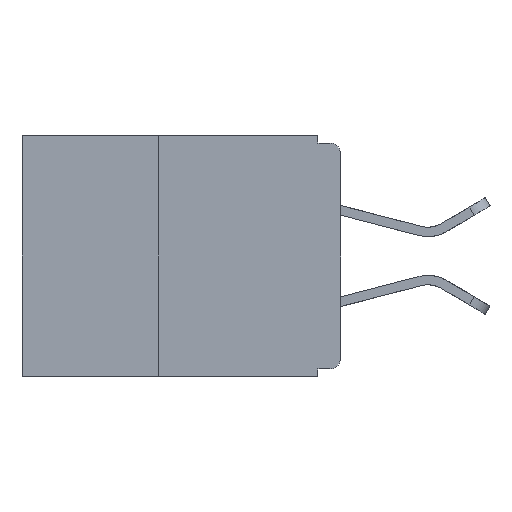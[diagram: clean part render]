
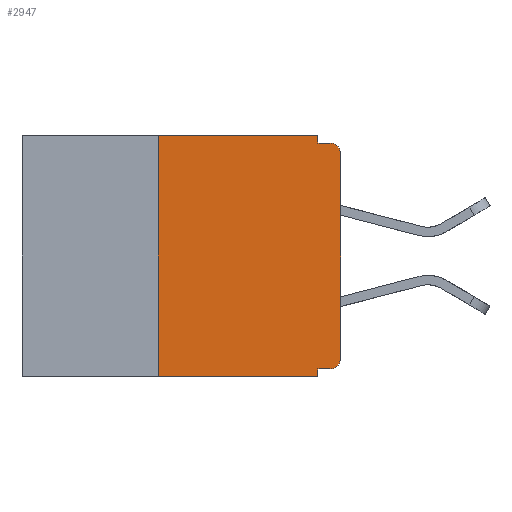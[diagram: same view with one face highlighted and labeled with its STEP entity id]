
A CAD part, left-side view. The second image highlights one B-rep face of the part: STEP entity #2947.
In plain terms, the highlighted planar face has unit normal (-1, 0, 0).
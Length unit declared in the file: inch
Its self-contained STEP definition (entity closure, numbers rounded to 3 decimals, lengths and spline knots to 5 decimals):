
#9 = VERTEX_POINT ( 'NONE', #16477 ) ;
#71 = DIRECTION ( 'NONE',  ( 0., 0., 1. ) ) ;
#332 = VERTEX_POINT ( 'NONE', #25629 ) ;
#1171 = CARTESIAN_POINT ( 'NONE',  ( 0., 0.25, -0.33 ) ) ;
#1781 = VERTEX_POINT ( 'NONE', #1171 ) ;
#1976 = DIRECTION ( 'NONE',  ( 0., 1., 0. ) ) ;
#2089 = CARTESIAN_POINT ( 'NONE',  ( 0., 0.031, -0.33 ) ) ;
#2160 = DIRECTION ( 'NONE',  ( 0., -1., 0. ) ) ;
#2727 = ORIENTED_EDGE ( 'NONE', *, *, #24573, .T. ) ;
#2947 = ADVANCED_FACE ( 'NONE', ( #3473 ), #28532, .F. ) ;
#3438 = ORIENTED_EDGE ( 'NONE', *, *, #26705, .F. ) ;
#3473 = FACE_OUTER_BOUND ( 'NONE', #21040, .T. ) ;
#4271 = VECTOR ( 'NONE', #12993, 39.37008 ) ;
#4609 = DIRECTION ( 'NONE',  ( -1., 0., 0. ) ) ;
#4970 = CARTESIAN_POINT ( 'NONE',  ( 0., 0., -0.305 ) ) ;
#5694 = VERTEX_POINT ( 'NONE', #16619 ) ;
#5990 = CARTESIAN_POINT ( 'NONE',  ( 0., 0.015, -0.305 ) ) ;
#5992 = CIRCLE ( 'NONE', #16226, 0.015 ) ;
#6116 = CARTESIAN_POINT ( 'NONE',  ( 0., 0.031, -0.32 ) ) ;
#6740 = LINE ( 'NONE', #29472, #19050 ) ;
#6777 = CARTESIAN_POINT ( 'NONE',  ( 0., 0., -0.01 ) ) ;
#7047 = CARTESIAN_POINT ( 'NONE',  ( 0., 0.015, -0.32 ) ) ;
#7069 = CARTESIAN_POINT ( 'NONE',  ( 0., 0., 0. ) ) ;
#8154 = LINE ( 'NONE', #6777, #14320 ) ;
#8337 = DIRECTION ( 'NONE',  ( 0., 0., -1. ) ) ;
#8576 = CARTESIAN_POINT ( 'NONE',  ( 0., 0.031, 0. ) ) ;
#9478 = EDGE_CURVE ( 'NONE', #10132, #332, #29723, .T. ) ;
#9685 = VECTOR ( 'NONE', #21821, 39.37008 ) ;
#9970 = EDGE_CURVE ( 'NONE', #5694, #20457, #16315, .T. ) ;
#10000 = AXIS2_PLACEMENT_3D ( 'NONE', #28494, #28205, #28182 ) ;
#10132 = VERTEX_POINT ( 'NONE', #23014 ) ;
#10174 = VERTEX_POINT ( 'NONE', #7047 ) ;
#10511 = LINE ( 'NONE', #13828, #11231 ) ;
#10670 = CARTESIAN_POINT ( 'NONE',  ( 0., 0.031, -0.33 ) ) ;
#11231 = VECTOR ( 'NONE', #2160, 39.37008 ) ;
#11484 = DIRECTION ( 'NONE',  ( 0., -1., 0. ) ) ;
#11510 = ORIENTED_EDGE ( 'NONE', *, *, #9970, .F. ) ;
#11711 = EDGE_CURVE ( 'NONE', #12384, #14481, #22667, .T. ) ;
#12384 = VERTEX_POINT ( 'NONE', #6116 ) ;
#12535 = CARTESIAN_POINT ( 'NONE',  ( 0., 0.25, -0.33 ) ) ;
#12993 = DIRECTION ( 'NONE',  ( 0., 0., -1. ) ) ;
#13828 = CARTESIAN_POINT ( 'NONE',  ( 0., 0.437, -0.33 ) ) ;
#14320 = VECTOR ( 'NONE', #11484, 39.37008 ) ;
#14481 = VERTEX_POINT ( 'NONE', #2089 ) ;
#15459 = ORIENTED_EDGE ( 'NONE', *, *, #17662, .F. ) ;
#15551 = DIRECTION ( 'NONE',  ( 0., -1., 0. ) ) ;
#16226 = AXIS2_PLACEMENT_3D ( 'NONE', #5990, #22083, #8337 ) ;
#16315 = LINE ( 'NONE', #24604, #27647 ) ;
#16477 = CARTESIAN_POINT ( 'NONE',  ( 0., 0.031, -0.01 ) ) ;
#16540 = ORIENTED_EDGE ( 'NONE', *, *, #27097, .T. ) ;
#16619 = CARTESIAN_POINT ( 'NONE',  ( 0., 0.25, 0. ) ) ;
#16702 = EDGE_CURVE ( 'NONE', #20457, #9, #21864, .T. ) ;
#16846 = VECTOR ( 'NONE', #19518, 39.37008 ) ;
#17314 = EDGE_CURVE ( 'NONE', #1781, #5694, #28858, .T. ) ;
#17610 = ORIENTED_EDGE ( 'NONE', *, *, #17314, .F. ) ;
#17662 = EDGE_CURVE ( 'NONE', #9, #332, #8154, .T. ) ;
#18415 = AXIS2_PLACEMENT_3D ( 'NONE', #18499, #4609, #20763 ) ;
#18499 = CARTESIAN_POINT ( 'NONE',  ( 0., 0.015, -0.025 ) ) ;
#19050 = VECTOR ( 'NONE', #1976, 39.37008 ) ;
#19518 = DIRECTION ( 'NONE',  ( 0., 0., 1. ) ) ;
#20243 = LINE ( 'NONE', #7069, #25563 ) ;
#20457 = VERTEX_POINT ( 'NONE', #8576 ) ;
#20763 = DIRECTION ( 'NONE',  ( 0., 0., -1. ) ) ;
#21040 = EDGE_LOOP ( 'NONE', ( #26099, #26790, #15459, #22220, #11510, #17610, #2727, #21182, #3438, #16540 ) ) ;
#21182 = ORIENTED_EDGE ( 'NONE', *, *, #11711, .F. ) ;
#21821 = DIRECTION ( 'NONE',  ( 0., 0., -1. ) ) ;
#21864 = LINE ( 'NONE', #28514, #9685 ) ;
#22083 = DIRECTION ( 'NONE',  ( -1., 0., 0. ) ) ;
#22220 = ORIENTED_EDGE ( 'NONE', *, *, #16702, .F. ) ;
#22667 = LINE ( 'NONE', #10670, #4271 ) ;
#23014 = CARTESIAN_POINT ( 'NONE',  ( 0., 0., -0.025 ) ) ;
#23532 = EDGE_CURVE ( 'NONE', #28603, #10132, #20243, .T. ) ;
#24573 = EDGE_CURVE ( 'NONE', #1781, #14481, #10511, .T. ) ;
#24604 = CARTESIAN_POINT ( 'NONE',  ( 0., 0.437, 0. ) ) ;
#25563 = VECTOR ( 'NONE', #71, 39.37008 ) ;
#25629 = CARTESIAN_POINT ( 'NONE',  ( 0., 0.015, -0.01 ) ) ;
#26099 = ORIENTED_EDGE ( 'NONE', *, *, #23532, .T. ) ;
#26705 = EDGE_CURVE ( 'NONE', #10174, #12384, #6740, .T. ) ;
#26790 = ORIENTED_EDGE ( 'NONE', *, *, #9478, .T. ) ;
#27097 = EDGE_CURVE ( 'NONE', #10174, #28603, #5992, .T. ) ;
#27647 = VECTOR ( 'NONE', #15551, 39.37008 ) ;
#28182 = DIRECTION ( 'NONE',  ( 0., 0., -1. ) ) ;
#28205 = DIRECTION ( 'NONE',  ( 1., 0., 0. ) ) ;
#28494 = CARTESIAN_POINT ( 'NONE',  ( 0., 0.437, 0. ) ) ;
#28514 = CARTESIAN_POINT ( 'NONE',  ( 0., 0.031, 0. ) ) ;
#28532 = PLANE ( 'NONE',  #10000 ) ;
#28603 = VERTEX_POINT ( 'NONE', #4970 ) ;
#28858 = LINE ( 'NONE', #12535, #16846 ) ;
#29472 = CARTESIAN_POINT ( 'NONE',  ( 0., 0., -0.32 ) ) ;
#29723 = CIRCLE ( 'NONE', #18415, 0.015 ) ;
